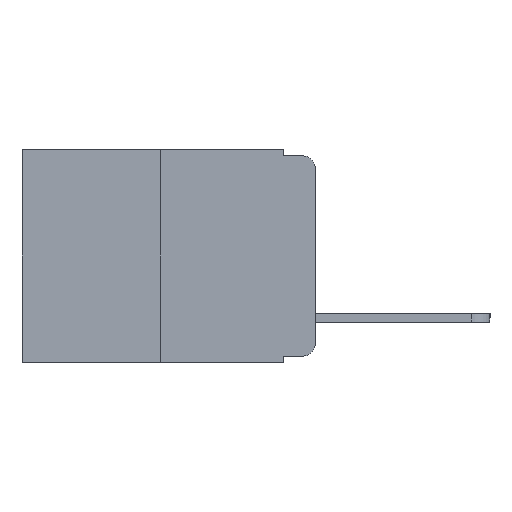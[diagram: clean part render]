
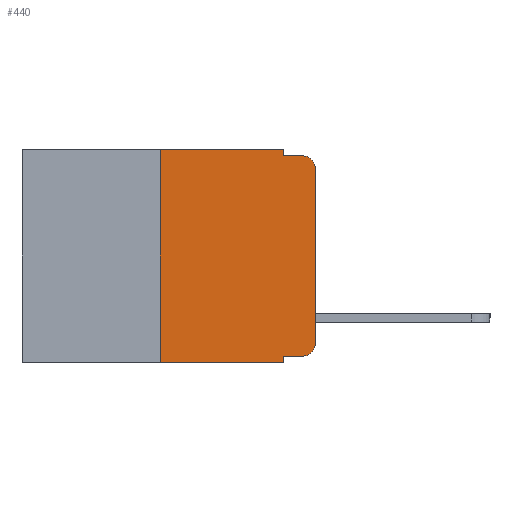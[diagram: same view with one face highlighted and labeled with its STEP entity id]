
A CAD part, left-side view. The second image highlights one B-rep face of the part: STEP entity #440.
In plain terms, the highlighted planar face has unit normal (-1, 0, 0).
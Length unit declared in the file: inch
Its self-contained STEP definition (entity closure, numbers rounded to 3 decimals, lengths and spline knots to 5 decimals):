
#43 = LINE ( 'NONE', #11766, #3672 ) ;
#301 = VECTOR ( 'NONE', #5465, 39.37008 ) ;
#314 = VERTEX_POINT ( 'NONE', #5937 ) ;
#440 = ADVANCED_FACE ( 'NONE', ( #9935 ), #10936, .F. ) ;
#524 = CIRCLE ( 'NONE', #5788, 0.02 ) ;
#730 = AXIS2_PLACEMENT_3D ( 'NONE', #1156, #9692, #2494 ) ;
#751 = LINE ( 'NONE', #6671, #9415 ) ;
#1139 = VERTEX_POINT ( 'NONE', #6514 ) ;
#1156 = CARTESIAN_POINT ( 'NONE',  ( 0., 0.02, -0.03 ) ) ;
#1384 = LINE ( 'NONE', #5709, #13036 ) ;
#1592 = AXIS2_PLACEMENT_3D ( 'NONE', #11582, #11424, #11680 ) ;
#1607 = LINE ( 'NONE', #12711, #13193 ) ;
#1800 = VECTOR ( 'NONE', #5278, 39.37008 ) ;
#2432 = ORIENTED_EDGE ( 'NONE', *, *, #2740, .F. ) ;
#2494 = DIRECTION ( 'NONE',  ( 0., 0., -1. ) ) ;
#2740 = EDGE_CURVE ( 'NONE', #13746, #4280, #1384, .T. ) ;
#2860 = ORIENTED_EDGE ( 'NONE', *, *, #5009, .T. ) ;
#3340 = CARTESIAN_POINT ( 'NONE',  ( 0., 0.25, 0. ) ) ;
#3478 = CIRCLE ( 'NONE', #730, 0.02 ) ;
#3672 = VECTOR ( 'NONE', #13778, 39.37008 ) ;
#3892 = ORIENTED_EDGE ( 'NONE', *, *, #5476, .T. ) ;
#4207 = CARTESIAN_POINT ( 'NONE',  ( 0., 0.051, 0. ) ) ;
#4280 = VERTEX_POINT ( 'NONE', #4207 ) ;
#4315 = ORIENTED_EDGE ( 'NONE', *, *, #5570, .T. ) ;
#4519 = VERTEX_POINT ( 'NONE', #4974 ) ;
#4974 = CARTESIAN_POINT ( 'NONE',  ( 0., 0.25, -0.343 ) ) ;
#5009 = EDGE_CURVE ( 'NONE', #9035, #314, #524, .T. ) ;
#5026 = CARTESIAN_POINT ( 'NONE',  ( 0., 0.051, -0.01 ) ) ;
#5047 = DIRECTION ( 'NONE',  ( -1., 0., 0. ) ) ;
#5168 = EDGE_CURVE ( 'NONE', #9800, #7650, #10127, .T. ) ;
#5188 = EDGE_CURVE ( 'NONE', #9800, #9035, #751, .T. ) ;
#5278 = DIRECTION ( 'NONE',  ( 0., 0., 1. ) ) ;
#5330 = EDGE_CURVE ( 'NONE', #4519, #13746, #6244, .T. ) ;
#5427 = EDGE_CURVE ( 'NONE', #4280, #7642, #1607, .T. ) ;
#5451 = EDGE_CURVE ( 'NONE', #7642, #1139, #12885, .T. ) ;
#5465 = DIRECTION ( 'NONE',  ( 0., 0., -1. ) ) ;
#5476 = EDGE_CURVE ( 'NONE', #12167, #1139, #3478, .T. ) ;
#5570 = EDGE_CURVE ( 'NONE', #314, #12167, #10960, .T. ) ;
#5612 = EDGE_CURVE ( 'NONE', #4519, #7650, #43, .T. ) ;
#5709 = CARTESIAN_POINT ( 'NONE',  ( 0., 0.473, 0. ) ) ;
#5788 = AXIS2_PLACEMENT_3D ( 'NONE', #11779, #5047, #12811 ) ;
#5878 = ORIENTED_EDGE ( 'NONE', *, *, #5168, .F. ) ;
#5937 = CARTESIAN_POINT ( 'NONE',  ( 0., 0., -0.313 ) ) ;
#6244 = LINE ( 'NONE', #3340, #14447 ) ;
#6260 = DIRECTION ( 'NONE',  ( 0., -1., 0. ) ) ;
#6514 = CARTESIAN_POINT ( 'NONE',  ( 0., 0.02, -0.01 ) ) ;
#6671 = CARTESIAN_POINT ( 'NONE',  ( 0., 0.051, -0.333 ) ) ;
#7041 = DIRECTION ( 'NONE',  ( 0., 0., 1. ) ) ;
#7112 = ORIENTED_EDGE ( 'NONE', *, *, #5427, .F. ) ;
#7642 = VERTEX_POINT ( 'NONE', #13482 ) ;
#7650 = VERTEX_POINT ( 'NONE', #14545 ) ;
#8535 = EDGE_LOOP ( 'NONE', ( #4315, #3892, #9757, #7112, #2432, #13821, #9597, #5878, #11776, #2860 ) ) ;
#8805 = CARTESIAN_POINT ( 'NONE',  ( 0., 0., 0. ) ) ;
#9035 = VERTEX_POINT ( 'NONE', #10298 ) ;
#9157 = DIRECTION ( 'NONE',  ( 0., -1., 0. ) ) ;
#9415 = VECTOR ( 'NONE', #13189, 39.37008 ) ;
#9597 = ORIENTED_EDGE ( 'NONE', *, *, #5612, .T. ) ;
#9607 = CARTESIAN_POINT ( 'NONE',  ( 0., 0.25, 0. ) ) ;
#9692 = DIRECTION ( 'NONE',  ( -1., 0., 0. ) ) ;
#9757 = ORIENTED_EDGE ( 'NONE', *, *, #5451, .F. ) ;
#9800 = VERTEX_POINT ( 'NONE', #10159 ) ;
#9935 = FACE_OUTER_BOUND ( 'NONE', #8535, .T. ) ;
#10127 = LINE ( 'NONE', #13142, #301 ) ;
#10159 = CARTESIAN_POINT ( 'NONE',  ( 0., 0.051, -0.333 ) ) ;
#10298 = CARTESIAN_POINT ( 'NONE',  ( 0., 0.02, -0.333 ) ) ;
#10936 = PLANE ( 'NONE',  #1592 ) ;
#10960 = LINE ( 'NONE', #8805, #1800 ) ;
#11424 = DIRECTION ( 'NONE',  ( 1., 0., 0. ) ) ;
#11582 = CARTESIAN_POINT ( 'NONE',  ( 0., 0.473, 0. ) ) ;
#11680 = DIRECTION ( 'NONE',  ( 0., 0., -1. ) ) ;
#11766 = CARTESIAN_POINT ( 'NONE',  ( 0., 0.473, -0.343 ) ) ;
#11776 = ORIENTED_EDGE ( 'NONE', *, *, #5188, .T. ) ;
#11779 = CARTESIAN_POINT ( 'NONE',  ( 0., 0.02, -0.313 ) ) ;
#12167 = VERTEX_POINT ( 'NONE', #13675 ) ;
#12576 = VECTOR ( 'NONE', #6260, 39.37008 ) ;
#12711 = CARTESIAN_POINT ( 'NONE',  ( 0., 0.051, 0. ) ) ;
#12811 = DIRECTION ( 'NONE',  ( 0., 0., -1. ) ) ;
#12885 = LINE ( 'NONE', #5026, #12576 ) ;
#13036 = VECTOR ( 'NONE', #9157, 39.37008 ) ;
#13142 = CARTESIAN_POINT ( 'NONE',  ( 0., 0.051, 0. ) ) ;
#13189 = DIRECTION ( 'NONE',  ( 0., -1., 0. ) ) ;
#13193 = VECTOR ( 'NONE', #14668, 39.37008 ) ;
#13482 = CARTESIAN_POINT ( 'NONE',  ( 0., 0.051, -0.01 ) ) ;
#13675 = CARTESIAN_POINT ( 'NONE',  ( 0., 0., -0.03 ) ) ;
#13746 = VERTEX_POINT ( 'NONE', #9607 ) ;
#13778 = DIRECTION ( 'NONE',  ( 0., -1., 0. ) ) ;
#13821 = ORIENTED_EDGE ( 'NONE', *, *, #5330, .F. ) ;
#14447 = VECTOR ( 'NONE', #7041, 39.37008 ) ;
#14545 = CARTESIAN_POINT ( 'NONE',  ( 0., 0.051, -0.343 ) ) ;
#14668 = DIRECTION ( 'NONE',  ( 0., 0., -1. ) ) ;
